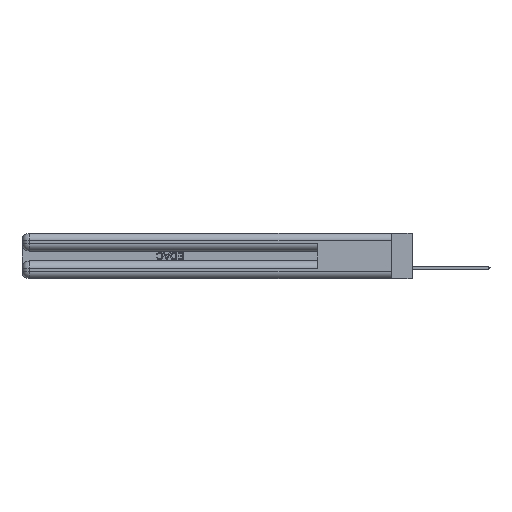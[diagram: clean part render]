
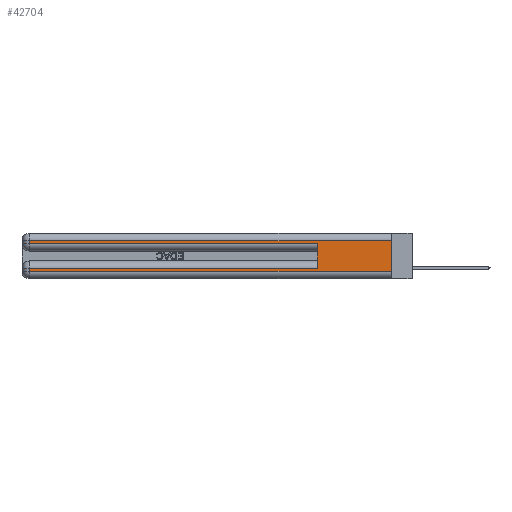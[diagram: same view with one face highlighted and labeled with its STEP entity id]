
A CAD part, left-side view. The second image highlights one B-rep face of the part: STEP entity #42704.
In plain terms, the highlighted planar face has unit normal (-1, 0, 0).
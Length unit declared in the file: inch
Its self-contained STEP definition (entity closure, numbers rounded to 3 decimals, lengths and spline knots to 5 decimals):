
#82 = LINE ( 'NONE', #19319, #31429 ) ;
#904 = LINE ( 'NONE', #14273, #18362 ) ;
#1080 = DIRECTION ( 'NONE',  ( 0., 0., -1. ) ) ;
#3529 = EDGE_CURVE ( 'NONE', #34924, #53717, #17793, .T. ) ;
#5966 = CARTESIAN_POINT ( 'NONE',  ( 0., 2.94, 0.37 ) ) ;
#6128 = EDGE_CURVE ( 'NONE', #51011, #42610, #52458, .T. ) ;
#6146 = DIRECTION ( 'NONE',  ( 0., 0., -1. ) ) ;
#7386 = CARTESIAN_POINT ( 'NONE',  ( 0., 2.94, 0.37 ) ) ;
#7502 = ORIENTED_EDGE ( 'NONE', *, *, #9087, .T. ) ;
#7957 = EDGE_CURVE ( 'NONE', #16554, #19215, #82, .T. ) ;
#9087 = EDGE_CURVE ( 'NONE', #24039, #19215, #21384, .T. ) ;
#10195 = LINE ( 'NONE', #5966, #54468 ) ;
#10330 = CARTESIAN_POINT ( 'NONE',  ( 0., 2.94, 0.06 ) ) ;
#10707 = ORIENTED_EDGE ( 'NONE', *, *, #13922, .T. ) ;
#11426 = VERTEX_POINT ( 'NONE', #15057 ) ;
#12371 = VECTOR ( 'NONE', #24279, 39.37008 ) ;
#12510 = ORIENTED_EDGE ( 'NONE', *, *, #7957, .F. ) ;
#13922 = EDGE_CURVE ( 'NONE', #16554, #11426, #48967, .T. ) ;
#14273 = CARTESIAN_POINT ( 'NONE',  ( 0., 0., 0.37 ) ) ;
#14918 = CARTESIAN_POINT ( 'NONE',  ( 0., 0.6, 0.085 ) ) ;
#15057 = CARTESIAN_POINT ( 'NONE',  ( 0., 2.94, 0.085 ) ) ;
#15541 = DIRECTION ( 'NONE',  ( 0., 1., 0. ) ) ;
#16554 = VERTEX_POINT ( 'NONE', #14918 ) ;
#17322 = EDGE_CURVE ( 'NONE', #11426, #51011, #54882, .T. ) ;
#17793 = LINE ( 'NONE', #53524, #24488 ) ;
#18362 = VECTOR ( 'NONE', #49665, 39.37008 ) ;
#19215 = VERTEX_POINT ( 'NONE', #49094 ) ;
#19319 = CARTESIAN_POINT ( 'NONE',  ( 0., 0.6, 0.145 ) ) ;
#19572 = CARTESIAN_POINT ( 'NONE',  ( 0., 2.94, 0.31 ) ) ;
#21384 = LINE ( 'NONE', #43213, #24708 ) ;
#22333 = CARTESIAN_POINT ( 'NONE',  ( 0., 0., 0.31 ) ) ;
#22339 = EDGE_CURVE ( 'NONE', #34924, #42610, #904, .T. ) ;
#23200 = DIRECTION ( 'NONE',  ( 0., 0., 1. ) ) ;
#24039 = VERTEX_POINT ( 'NONE', #28666 ) ;
#24279 = DIRECTION ( 'NONE',  ( 0., -1., 0. ) ) ;
#24488 = VECTOR ( 'NONE', #15541, 39.37008 ) ;
#24708 = VECTOR ( 'NONE', #43562, 39.37008 ) ;
#26372 = CARTESIAN_POINT ( 'NONE',  ( 0., 0., 0.37 ) ) ;
#28644 = ORIENTED_EDGE ( 'NONE', *, *, #6128, .T. ) ;
#28666 = CARTESIAN_POINT ( 'NONE',  ( 0., 2.94, 0.285 ) ) ;
#28743 = CARTESIAN_POINT ( 'NONE',  ( 0., 0., 0.06 ) ) ;
#28772 = DIRECTION ( 'NONE',  ( 0., 1., 0. ) ) ;
#29793 = CARTESIAN_POINT ( 'NONE',  ( 0., 0., 0.06 ) ) ;
#30487 = PLANE ( 'NONE',  #49936 ) ;
#31010 = DIRECTION ( 'NONE',  ( 1., 0., 0. ) ) ;
#31429 = VECTOR ( 'NONE', #23200, 39.37008 ) ;
#31789 = FACE_OUTER_BOUND ( 'NONE', #46132, .T. ) ;
#33453 = CARTESIAN_POINT ( 'NONE',  ( 0., 0., 0.085 ) ) ;
#34050 = VECTOR ( 'NONE', #54890, 39.37008 ) ;
#34924 = VERTEX_POINT ( 'NONE', #22333 ) ;
#36073 = EDGE_CURVE ( 'NONE', #53717, #24039, #10195, .T. ) ;
#37588 = VECTOR ( 'NONE', #28772, 39.37008 ) ;
#39140 = ORIENTED_EDGE ( 'NONE', *, *, #3529, .T. ) ;
#42610 = VERTEX_POINT ( 'NONE', #29793 ) ;
#42704 = ADVANCED_FACE ( 'NONE', ( #31789 ), #30487, .F. ) ;
#43213 = CARTESIAN_POINT ( 'NONE',  ( 0., 0., 0.285 ) ) ;
#43562 = DIRECTION ( 'NONE',  ( 0., -1., 0. ) ) ;
#45789 = ORIENTED_EDGE ( 'NONE', *, *, #36073, .T. ) ;
#46132 = EDGE_LOOP ( 'NONE', ( #50783, #39140, #45789, #7502, #12510, #10707, #52620, #28644 ) ) ;
#48967 = LINE ( 'NONE', #33453, #37588 ) ;
#49094 = CARTESIAN_POINT ( 'NONE',  ( 0., 0.6, 0.285 ) ) ;
#49665 = DIRECTION ( 'NONE',  ( 0., 0., -1. ) ) ;
#49936 = AXIS2_PLACEMENT_3D ( 'NONE', #26372, #31010, #1080 ) ;
#50783 = ORIENTED_EDGE ( 'NONE', *, *, #22339, .F. ) ;
#51011 = VERTEX_POINT ( 'NONE', #10330 ) ;
#52458 = LINE ( 'NONE', #28743, #12371 ) ;
#52620 = ORIENTED_EDGE ( 'NONE', *, *, #17322, .T. ) ;
#53524 = CARTESIAN_POINT ( 'NONE',  ( 0., 0., 0.31 ) ) ;
#53717 = VERTEX_POINT ( 'NONE', #19572 ) ;
#54468 = VECTOR ( 'NONE', #6146, 39.37008 ) ;
#54882 = LINE ( 'NONE', #7386, #34050 ) ;
#54890 = DIRECTION ( 'NONE',  ( 0., 0., -1. ) ) ;
